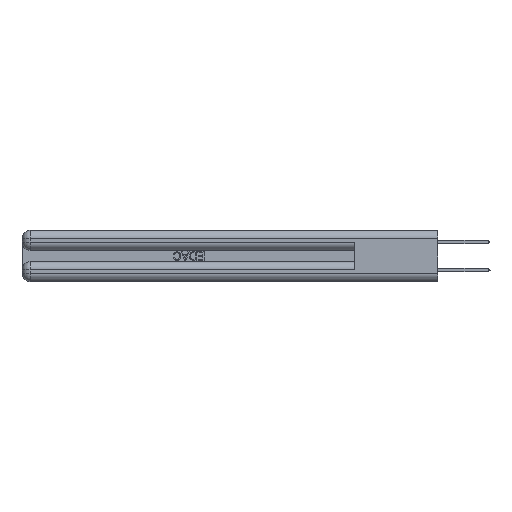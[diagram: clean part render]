
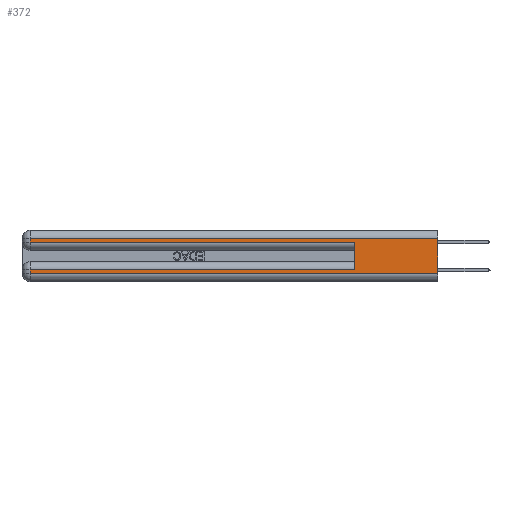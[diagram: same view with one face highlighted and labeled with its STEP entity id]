
A CAD part, left-side view. The second image highlights one B-rep face of the part: STEP entity #372.
In plain terms, the highlighted planar face has unit normal (-1, 0, 0).
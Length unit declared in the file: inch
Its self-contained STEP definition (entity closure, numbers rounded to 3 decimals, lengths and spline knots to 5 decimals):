
#372 = ADVANCED_FACE ( 'NONE', ( #19970 ), #28607, .F. ) ;
#1033 = VERTEX_POINT ( 'NONE', #15741 ) ;
#1352 = CARTESIAN_POINT ( 'NONE',  ( 0., 0.6, 0.285 ) ) ;
#1874 = LINE ( 'NONE', #23624, #37433 ) ;
#2355 = AXIS2_PLACEMENT_3D ( 'NONE', #39117, #7282, #32160 ) ;
#2384 = CARTESIAN_POINT ( 'NONE',  ( 0., 2.94, 0.37 ) ) ;
#2421 = CARTESIAN_POINT ( 'NONE',  ( 0., 0.6, 0.145 ) ) ;
#2925 = DIRECTION ( 'NONE',  ( 0., 1., 0. ) ) ;
#3099 = EDGE_LOOP ( 'NONE', ( #5349, #28104, #30098, #43460, #6746, #15687, #4296, #36821 ) ) ;
#4296 = ORIENTED_EDGE ( 'NONE', *, *, #18947, .T. ) ;
#4299 = VERTEX_POINT ( 'NONE', #31812 ) ;
#5349 = ORIENTED_EDGE ( 'NONE', *, *, #32666, .F. ) ;
#6660 = VECTOR ( 'NONE', #36567, 39.37008 ) ;
#6746 = ORIENTED_EDGE ( 'NONE', *, *, #25869, .F. ) ;
#7282 = DIRECTION ( 'NONE',  ( 1., 0., 0. ) ) ;
#7379 = CARTESIAN_POINT ( 'NONE',  ( 0., 2.94, 0.085 ) ) ;
#9464 = DIRECTION ( 'NONE',  ( 0., -1., 0. ) ) ;
#9706 = VECTOR ( 'NONE', #20166, 39.37008 ) ;
#10200 = VERTEX_POINT ( 'NONE', #7379 ) ;
#10839 = LINE ( 'NONE', #2421, #9706 ) ;
#12014 = VECTOR ( 'NONE', #42541, 39.37008 ) ;
#14023 = CARTESIAN_POINT ( 'NONE',  ( 0., 2.94, 0.37 ) ) ;
#15162 = VERTEX_POINT ( 'NONE', #1352 ) ;
#15687 = ORIENTED_EDGE ( 'NONE', *, *, #27746, .T. ) ;
#15741 = CARTESIAN_POINT ( 'NONE',  ( 0., 2.94, 0.06 ) ) ;
#17788 = VECTOR ( 'NONE', #24581, 39.37008 ) ;
#18115 = VECTOR ( 'NONE', #45058, 39.37008 ) ;
#18464 = DIRECTION ( 'NONE',  ( 0., 1., 0. ) ) ;
#18947 = EDGE_CURVE ( 'NONE', #10200, #1033, #27520, .T. ) ;
#19607 = EDGE_CURVE ( 'NONE', #1033, #24111, #1874, .T. ) ;
#19970 = FACE_OUTER_BOUND ( 'NONE', #3099, .T. ) ;
#20166 = DIRECTION ( 'NONE',  ( 0., 0., 1. ) ) ;
#20659 = CARTESIAN_POINT ( 'NONE',  ( 0., 0., 0.085 ) ) ;
#22308 = CARTESIAN_POINT ( 'NONE',  ( 0., 0., 0.37 ) ) ;
#22899 = LINE ( 'NONE', #20659, #40641 ) ;
#23268 = CARTESIAN_POINT ( 'NONE',  ( 0., 0., 0.31 ) ) ;
#23624 = CARTESIAN_POINT ( 'NONE',  ( 0., 0., 0.06 ) ) ;
#24111 = VERTEX_POINT ( 'NONE', #31780 ) ;
#24581 = DIRECTION ( 'NONE',  ( 0., 0., -1. ) ) ;
#25869 = EDGE_CURVE ( 'NONE', #44773, #15162, #10839, .T. ) ;
#27520 = LINE ( 'NONE', #2384, #18115 ) ;
#27746 = EDGE_CURVE ( 'NONE', #44773, #10200, #22899, .T. ) ;
#27915 = VERTEX_POINT ( 'NONE', #39398 ) ;
#28104 = ORIENTED_EDGE ( 'NONE', *, *, #28615, .T. ) ;
#28314 = CARTESIAN_POINT ( 'NONE',  ( 0., 0., 0.285 ) ) ;
#28329 = LINE ( 'NONE', #14023, #17788 ) ;
#28607 = PLANE ( 'NONE',  #2355 ) ;
#28615 = EDGE_CURVE ( 'NONE', #32165, #4299, #43887, .T. ) ;
#30098 = ORIENTED_EDGE ( 'NONE', *, *, #34030, .T. ) ;
#31780 = CARTESIAN_POINT ( 'NONE',  ( 0., 0., 0.06 ) ) ;
#31812 = CARTESIAN_POINT ( 'NONE',  ( 0., 2.94, 0.31 ) ) ;
#32160 = DIRECTION ( 'NONE',  ( 0., 0., -1. ) ) ;
#32165 = VERTEX_POINT ( 'NONE', #23268 ) ;
#32666 = EDGE_CURVE ( 'NONE', #32165, #24111, #45533, .T. ) ;
#34030 = EDGE_CURVE ( 'NONE', #4299, #27915, #28329, .T. ) ;
#34568 = CARTESIAN_POINT ( 'NONE',  ( 0., 0.6, 0.085 ) ) ;
#36567 = DIRECTION ( 'NONE',  ( 0., 0., -1. ) ) ;
#36821 = ORIENTED_EDGE ( 'NONE', *, *, #19607, .T. ) ;
#37433 = VECTOR ( 'NONE', #9464, 39.37008 ) ;
#39117 = CARTESIAN_POINT ( 'NONE',  ( 0., 0., 0.37 ) ) ;
#39398 = CARTESIAN_POINT ( 'NONE',  ( 0., 2.94, 0.285 ) ) ;
#39434 = EDGE_CURVE ( 'NONE', #27915, #15162, #40325, .T. ) ;
#40325 = LINE ( 'NONE', #28314, #12014 ) ;
#40641 = VECTOR ( 'NONE', #2925, 39.37008 ) ;
#42541 = DIRECTION ( 'NONE',  ( 0., -1., 0. ) ) ;
#42779 = VECTOR ( 'NONE', #18464, 39.37008 ) ;
#43217 = CARTESIAN_POINT ( 'NONE',  ( 0., 0., 0.31 ) ) ;
#43460 = ORIENTED_EDGE ( 'NONE', *, *, #39434, .T. ) ;
#43887 = LINE ( 'NONE', #43217, #42779 ) ;
#44773 = VERTEX_POINT ( 'NONE', #34568 ) ;
#45058 = DIRECTION ( 'NONE',  ( 0., 0., -1. ) ) ;
#45533 = LINE ( 'NONE', #22308, #6660 ) ;
